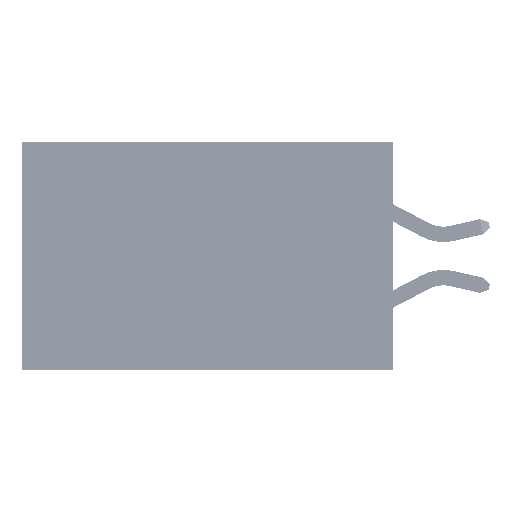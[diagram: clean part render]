
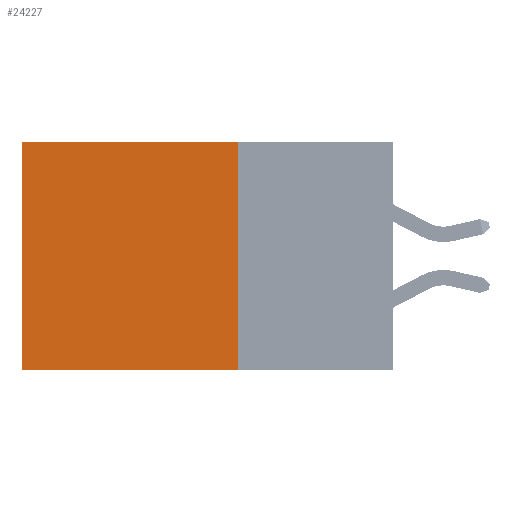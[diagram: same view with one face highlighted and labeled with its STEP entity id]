
A CAD part, left-side view. The second image highlights one B-rep face of the part: STEP entity #24227.
In plain terms, the highlighted planar face has unit normal (-1, 0, 0).
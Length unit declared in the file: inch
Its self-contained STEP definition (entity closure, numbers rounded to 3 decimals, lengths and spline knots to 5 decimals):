
#1726 = VERTEX_POINT ( 'NONE', #32906 ) ;
#2015 = CARTESIAN_POINT ( 'NONE',  ( 0.2875, 0.25, -0.37 ) ) ;
#2273 = VERTEX_POINT ( 'NONE', #30385 ) ;
#4339 = DIRECTION ( 'NONE',  ( 0., 1., 0. ) ) ;
#4526 = ORIENTED_EDGE ( 'NONE', *, *, #21054, .F. ) ;
#9351 = CARTESIAN_POINT ( 'NONE',  ( 0.2875, 0.25, -0.37 ) ) ;
#9692 = EDGE_CURVE ( 'NONE', #38390, #17415, #27091, .T. ) ;
#13769 = DIRECTION ( 'NONE',  ( 0., 0., -1. ) ) ;
#14768 = CARTESIAN_POINT ( 'NONE',  ( 0.2875, 0.25, 0. ) ) ;
#15828 = DIRECTION ( 'NONE',  ( 0., 0., -1. ) ) ;
#17415 = VERTEX_POINT ( 'NONE', #9351 ) ;
#19766 = PLANE ( 'NONE',  #21038 ) ;
#21038 = AXIS2_PLACEMENT_3D ( 'NONE', #27684, #31791, #15828 ) ;
#21054 = EDGE_CURVE ( 'NONE', #17415, #1726, #22006, .T. ) ;
#22006 = LINE ( 'NONE', #2015, #33622 ) ;
#22880 = ORIENTED_EDGE ( 'NONE', *, *, #26167, .T. ) ;
#23107 = CARTESIAN_POINT ( 'NONE',  ( 0.2875, 0.25, 0. ) ) ;
#24227 = ADVANCED_FACE ( 'NONE', ( #27317 ), #19766, .F. ) ;
#24769 = LINE ( 'NONE', #37235, #38880 ) ;
#26167 = EDGE_CURVE ( 'NONE', #38390, #2273, #41240, .T. ) ;
#27091 = LINE ( 'NONE', #14768, #31383 ) ;
#27317 = FACE_OUTER_BOUND ( 'NONE', #38220, .T. ) ;
#27684 = CARTESIAN_POINT ( 'NONE',  ( 0.2875, 0.25, 0. ) ) ;
#27863 = CARTESIAN_POINT ( 'NONE',  ( 0.2875, 0.25, 0. ) ) ;
#30385 = CARTESIAN_POINT ( 'NONE',  ( 0.2875, 0.6, 0. ) ) ;
#30554 = DIRECTION ( 'NONE',  ( 0., 0., -1. ) ) ;
#31383 = VECTOR ( 'NONE', #30554, 39.37008 ) ;
#31791 = DIRECTION ( 'NONE',  ( 1., 0., 0. ) ) ;
#32906 = CARTESIAN_POINT ( 'NONE',  ( 0.2875, 0.6, -0.37 ) ) ;
#33622 = VECTOR ( 'NONE', #37083, 39.37008 ) ;
#37083 = DIRECTION ( 'NONE',  ( 0., 1., 0. ) ) ;
#37235 = CARTESIAN_POINT ( 'NONE',  ( 0.2875, 0.6, 0. ) ) ;
#38220 = EDGE_LOOP ( 'NONE', ( #44538, #4526, #40328, #22880 ) ) ;
#38390 = VERTEX_POINT ( 'NONE', #23107 ) ;
#38867 = EDGE_CURVE ( 'NONE', #2273, #1726, #24769, .T. ) ;
#38880 = VECTOR ( 'NONE', #13769, 39.37008 ) ;
#40328 = ORIENTED_EDGE ( 'NONE', *, *, #9692, .F. ) ;
#41240 = LINE ( 'NONE', #27863, #48681 ) ;
#44538 = ORIENTED_EDGE ( 'NONE', *, *, #38867, .T. ) ;
#48681 = VECTOR ( 'NONE', #4339, 39.37008 ) ;
